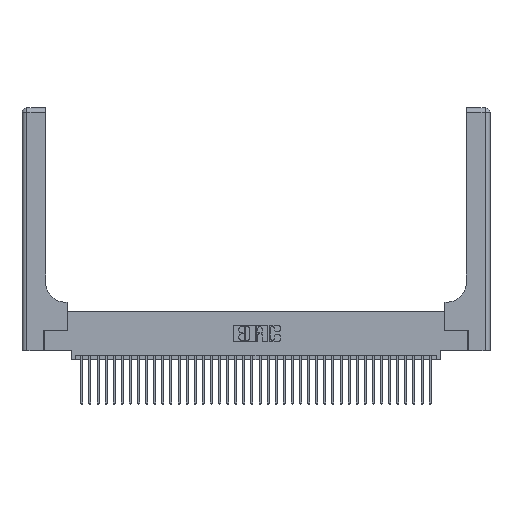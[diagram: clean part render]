
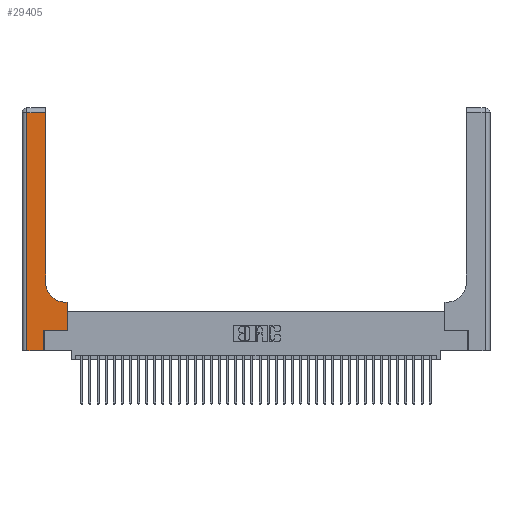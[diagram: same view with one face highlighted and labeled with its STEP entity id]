
A CAD part, top view. The second image highlights one B-rep face of the part: STEP entity #29405.
In plain terms, the highlighted planar face has unit normal (0, 0, 1).
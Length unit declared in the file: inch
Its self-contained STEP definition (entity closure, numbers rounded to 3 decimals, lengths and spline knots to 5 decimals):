
#74 = VECTOR ( 'NONE', #37332, 39.37008 ) ;
#1122 = DIRECTION ( 'NONE',  ( -1., 0., 0. ) ) ;
#2709 = DIRECTION ( 'NONE',  ( 1., 0., 0. ) ) ;
#2837 = LINE ( 'NONE', #26325, #10006 ) ;
#2897 = DIRECTION ( 'NONE',  ( 0., 1., 0. ) ) ;
#3252 = CARTESIAN_POINT ( 'NONE',  ( 0.2915, 2.94, 0.37 ) ) ;
#3493 = CARTESIAN_POINT ( 'NONE',  ( 0.2915, 0.6, 0.37 ) ) ;
#3690 = CARTESIAN_POINT ( 'NONE',  ( 0.06, 3., 0.37 ) ) ;
#4951 = DIRECTION ( 'NONE',  ( 0., 1., 0. ) ) ;
#5332 = EDGE_CURVE ( 'NONE', #5449, #11559, #29181, .T. ) ;
#5449 = VERTEX_POINT ( 'NONE', #34470 ) ;
#5506 = VERTEX_POINT ( 'NONE', #31677 ) ;
#6136 = AXIS2_PLACEMENT_3D ( 'NONE', #15732, #37078, #18799 ) ;
#6439 = CARTESIAN_POINT ( 'NONE',  ( 0.5585, 0.6, 0.37 ) ) ;
#6599 = VECTOR ( 'NONE', #2897, 39.37008 ) ;
#6707 = EDGE_LOOP ( 'NONE', ( #11634, #13769, #38058, #19937, #28091, #8468, #32413, #9507, #31210 ) ) ;
#7132 = EDGE_CURVE ( 'NONE', #39575, #14126, #20881, .T. ) ;
#7569 = LINE ( 'NONE', #17915, #39112 ) ;
#8242 = LINE ( 'NONE', #3690, #74 ) ;
#8468 = ORIENTED_EDGE ( 'NONE', *, *, #21519, .T. ) ;
#9507 = ORIENTED_EDGE ( 'NONE', *, *, #7132, .T. ) ;
#9510 = DIRECTION ( 'NONE',  ( -1., 0., 0. ) ) ;
#10006 = VECTOR ( 'NONE', #4951, 39.37008 ) ;
#10078 = VERTEX_POINT ( 'NONE', #27209 ) ;
#10256 = CARTESIAN_POINT ( 'NONE',  ( 0.269, 0., 0.37 ) ) ;
#10922 = DIRECTION ( 'NONE',  ( 0., 1., 0. ) ) ;
#11308 = CARTESIAN_POINT ( 'NONE',  ( 0.5585, 0.25, 0.37 ) ) ;
#11559 = VERTEX_POINT ( 'NONE', #10256 ) ;
#11634 = ORIENTED_EDGE ( 'NONE', *, *, #36964, .T. ) ;
#12132 = EDGE_CURVE ( 'NONE', #5506, #5449, #8242, .T. ) ;
#12755 = VECTOR ( 'NONE', #9510, 39.37008 ) ;
#13002 = FACE_OUTER_BOUND ( 'NONE', #6707, .T. ) ;
#13769 = ORIENTED_EDGE ( 'NONE', *, *, #20319, .T. ) ;
#13831 = LINE ( 'NONE', #38416, #30104 ) ;
#14126 = VERTEX_POINT ( 'NONE', #23763 ) ;
#14166 = LINE ( 'NONE', #39301, #29473 ) ;
#14757 = EDGE_CURVE ( 'NONE', #29659, #39575, #32904, .T. ) ;
#15732 = CARTESIAN_POINT ( 'NONE',  ( 0.5415, 0.85, 0.37 ) ) ;
#16401 = PLANE ( 'NONE',  #39360 ) ;
#17915 = CARTESIAN_POINT ( 'NONE',  ( 0., 2.94, 0.37 ) ) ;
#18279 = CARTESIAN_POINT ( 'NONE',  ( 0.5585, 0.25, 0.37 ) ) ;
#18799 = DIRECTION ( 'NONE',  ( 1., 0., 0. ) ) ;
#19255 = VERTEX_POINT ( 'NONE', #28027 ) ;
#19449 = DIRECTION ( 'NONE',  ( 0., 0., -1. ) ) ;
#19837 = VERTEX_POINT ( 'NONE', #3252 ) ;
#19937 = ORIENTED_EDGE ( 'NONE', *, *, #5332, .T. ) ;
#20319 = EDGE_CURVE ( 'NONE', #19837, #5506, #7569, .T. ) ;
#20881 = LINE ( 'NONE', #3493, #12755 ) ;
#21519 = EDGE_CURVE ( 'NONE', #19255, #29659, #14166, .T. ) ;
#23763 = CARTESIAN_POINT ( 'NONE',  ( 0.5415, 0.6, 0.37 ) ) ;
#26325 = CARTESIAN_POINT ( 'NONE',  ( 0.269, 0., 0.37 ) ) ;
#27209 = CARTESIAN_POINT ( 'NONE',  ( 0.2915, 0.85, 0.37 ) ) ;
#27819 = CARTESIAN_POINT ( 'NONE',  ( 0., 0., 0.37 ) ) ;
#28027 = CARTESIAN_POINT ( 'NONE',  ( 0.269, 0.25, 0.37 ) ) ;
#28091 = ORIENTED_EDGE ( 'NONE', *, *, #32204, .T. ) ;
#29181 = LINE ( 'NONE', #27819, #37274 ) ;
#29405 = ADVANCED_FACE ( 'NONE', ( #13002 ), #16401, .F. ) ;
#29473 = VECTOR ( 'NONE', #2709, 39.37008 ) ;
#29659 = VERTEX_POINT ( 'NONE', #11308 ) ;
#30104 = VECTOR ( 'NONE', #10922, 39.37008 ) ;
#30892 = DIRECTION ( 'NONE',  ( 1., 0., 0. ) ) ;
#31210 = ORIENTED_EDGE ( 'NONE', *, *, #31333, .T. ) ;
#31333 = EDGE_CURVE ( 'NONE', #14126, #10078, #37778, .T. ) ;
#31677 = CARTESIAN_POINT ( 'NONE',  ( 0.06, 2.94, 0.37 ) ) ;
#32204 = EDGE_CURVE ( 'NONE', #11559, #19255, #2837, .T. ) ;
#32413 = ORIENTED_EDGE ( 'NONE', *, *, #14757, .T. ) ;
#32904 = LINE ( 'NONE', #18279, #6599 ) ;
#34470 = CARTESIAN_POINT ( 'NONE',  ( 0.06, 0., 0.37 ) ) ;
#36321 = DIRECTION ( 'NONE',  ( -1., 0., 0. ) ) ;
#36964 = EDGE_CURVE ( 'NONE', #10078, #19837, #13831, .T. ) ;
#37078 = DIRECTION ( 'NONE',  ( 0., 0., -1. ) ) ;
#37274 = VECTOR ( 'NONE', #30892, 39.37008 ) ;
#37332 = DIRECTION ( 'NONE',  ( 0., -1., 0. ) ) ;
#37756 = CARTESIAN_POINT ( 'NONE',  ( 0., 3., 0.37 ) ) ;
#37778 = CIRCLE ( 'NONE', #6136, 0.25 ) ;
#38058 = ORIENTED_EDGE ( 'NONE', *, *, #12132, .T. ) ;
#38416 = CARTESIAN_POINT ( 'NONE',  ( 0.2915, 3., 0.37 ) ) ;
#39112 = VECTOR ( 'NONE', #36321, 39.37008 ) ;
#39301 = CARTESIAN_POINT ( 'NONE',  ( 0.269, 0.25, 0.37 ) ) ;
#39360 = AXIS2_PLACEMENT_3D ( 'NONE', #37756, #19449, #1122 ) ;
#39575 = VERTEX_POINT ( 'NONE', #6439 ) ;
